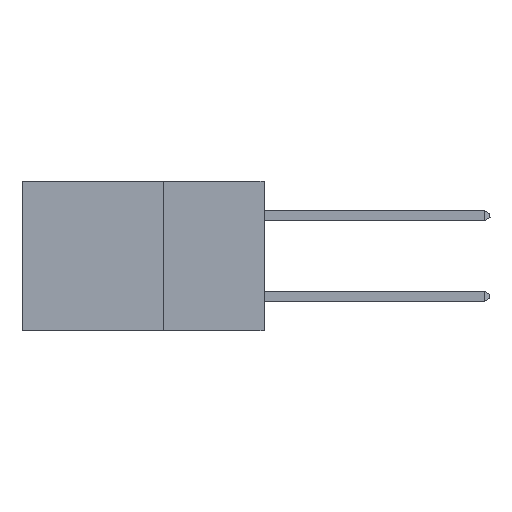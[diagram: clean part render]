
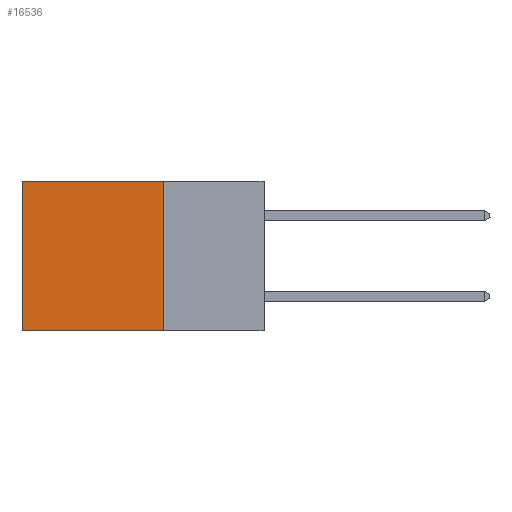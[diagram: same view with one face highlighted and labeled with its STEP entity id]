
A CAD part, left-side view. The second image highlights one B-rep face of the part: STEP entity #16536.
In plain terms, the highlighted planar face has unit normal (-1, 0, 0).
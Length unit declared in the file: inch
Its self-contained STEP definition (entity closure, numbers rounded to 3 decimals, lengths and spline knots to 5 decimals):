
#899 = EDGE_LOOP ( 'NONE', ( #6924, #18035, #7251, #18438 ) ) ;
#1310 = PLANE ( 'NONE',  #14220 ) ;
#1467 = DIRECTION ( 'NONE',  ( 0., 1., 0. ) ) ;
#1482 = EDGE_CURVE ( 'NONE', #18848, #2005, #12620, .T. ) ;
#2005 = VERTEX_POINT ( 'NONE', #18622 ) ;
#2259 = CARTESIAN_POINT ( 'NONE',  ( 0.298, 0.25, 0. ) ) ;
#4475 = CARTESIAN_POINT ( 'NONE',  ( 0.298, 0.25, 0. ) ) ;
#4806 = VERTEX_POINT ( 'NONE', #19669 ) ;
#4993 = VECTOR ( 'NONE', #10923, 39.37008 ) ;
#5352 = FACE_OUTER_BOUND ( 'NONE', #899, .T. ) ;
#5353 = LINE ( 'NONE', #6125, #12357 ) ;
#6076 = DIRECTION ( 'NONE',  ( 1., 0., 0. ) ) ;
#6125 = CARTESIAN_POINT ( 'NONE',  ( 0.298, 0.6, 0. ) ) ;
#6924 = ORIENTED_EDGE ( 'NONE', *, *, #14429, .T. ) ;
#6973 = LINE ( 'NONE', #18983, #4993 ) ;
#7251 = ORIENTED_EDGE ( 'NONE', *, *, #1482, .F. ) ;
#7331 = LINE ( 'NONE', #14040, #10086 ) ;
#8348 = VECTOR ( 'NONE', #12207, 39.37008 ) ;
#10086 = VECTOR ( 'NONE', #1467, 39.37008 ) ;
#10923 = DIRECTION ( 'NONE',  ( 0., 1., 0. ) ) ;
#11442 = EDGE_CURVE ( 'NONE', #2005, #4806, #6973, .T. ) ;
#11691 = CARTESIAN_POINT ( 'NONE',  ( 0.298, 0.25, 0. ) ) ;
#12207 = DIRECTION ( 'NONE',  ( 0., 0., -1. ) ) ;
#12357 = VECTOR ( 'NONE', #12731, 39.37008 ) ;
#12620 = LINE ( 'NONE', #2259, #8348 ) ;
#12731 = DIRECTION ( 'NONE',  ( 0., 0., -1. ) ) ;
#12868 = VERTEX_POINT ( 'NONE', #17765 ) ;
#14040 = CARTESIAN_POINT ( 'NONE',  ( 0.298, 0.25, 0. ) ) ;
#14156 = DIRECTION ( 'NONE',  ( 0., 0., -1. ) ) ;
#14220 = AXIS2_PLACEMENT_3D ( 'NONE', #4475, #6076, #14156 ) ;
#14429 = EDGE_CURVE ( 'NONE', #12868, #4806, #5353, .T. ) ;
#16536 = ADVANCED_FACE ( 'NONE', ( #5352 ), #1310, .F. ) ;
#16802 = EDGE_CURVE ( 'NONE', #18848, #12868, #7331, .T. ) ;
#17765 = CARTESIAN_POINT ( 'NONE',  ( 0.298, 0.6, 0. ) ) ;
#18035 = ORIENTED_EDGE ( 'NONE', *, *, #11442, .F. ) ;
#18438 = ORIENTED_EDGE ( 'NONE', *, *, #16802, .T. ) ;
#18622 = CARTESIAN_POINT ( 'NONE',  ( 0.298, 0.25, -0.37 ) ) ;
#18848 = VERTEX_POINT ( 'NONE', #11691 ) ;
#18983 = CARTESIAN_POINT ( 'NONE',  ( 0.298, 0.25, -0.37 ) ) ;
#19669 = CARTESIAN_POINT ( 'NONE',  ( 0.298, 0.6, -0.37 ) ) ;
